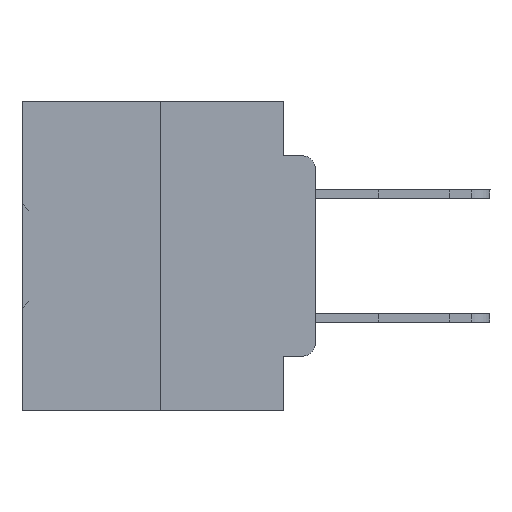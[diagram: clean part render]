
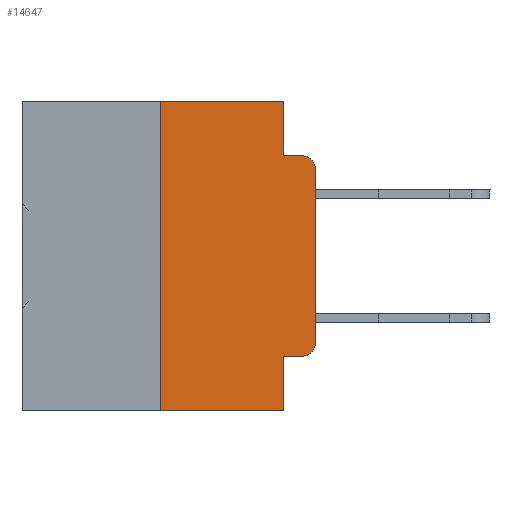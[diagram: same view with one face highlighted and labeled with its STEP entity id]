
A CAD part, left-side view. The second image highlights one B-rep face of the part: STEP entity #14647.
In plain terms, the highlighted planar face has unit normal (-1, 0, 0).
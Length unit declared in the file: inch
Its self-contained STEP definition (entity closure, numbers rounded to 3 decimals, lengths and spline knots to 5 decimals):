
#165 = ORIENTED_EDGE ( 'NONE', *, *, #10453, .F. ) ;
#388 = LINE ( 'NONE', #12724, #21902 ) ;
#482 = CARTESIAN_POINT ( 'NONE',  ( 0., 0.02, -0.3915 ) ) ;
#504 = EDGE_CURVE ( 'NONE', #18739, #6508, #18094, .T. ) ;
#889 = DIRECTION ( 'NONE',  ( 0., 0., -1. ) ) ;
#1047 = CARTESIAN_POINT ( 'NONE',  ( 0., 0.473, 0. ) ) ;
#1151 = VERTEX_POINT ( 'NONE', #35443 ) ;
#1273 = CARTESIAN_POINT ( 'NONE',  ( 0., 0.25, -0.5 ) ) ;
#1347 = VECTOR ( 'NONE', #1844, 39.37008 ) ;
#1844 = DIRECTION ( 'NONE',  ( 0., 0., 1. ) ) ;
#3006 = ORIENTED_EDGE ( 'NONE', *, *, #504, .T. ) ;
#3574 = VERTEX_POINT ( 'NONE', #27225 ) ;
#3698 = ORIENTED_EDGE ( 'NONE', *, *, #39091, .F. ) ;
#4231 = EDGE_CURVE ( 'NONE', #32129, #24944, #15705, .T. ) ;
#4873 = DIRECTION ( 'NONE',  ( 0., -1., 0. ) ) ;
#4876 = EDGE_CURVE ( 'NONE', #31318, #14479, #19327, .T. ) ;
#5025 = CARTESIAN_POINT ( 'NONE',  ( 0., 0., 0. ) ) ;
#5856 = DIRECTION ( 'NONE',  ( 0., 0., 1. ) ) ;
#6166 = ORIENTED_EDGE ( 'NONE', *, *, #20679, .T. ) ;
#6465 = VECTOR ( 'NONE', #28277, 39.37008 ) ;
#6508 = VERTEX_POINT ( 'NONE', #35220 ) ;
#6914 = LINE ( 'NONE', #37143, #18299 ) ;
#6916 = ORIENTED_EDGE ( 'NONE', *, *, #4231, .T. ) ;
#7059 = AXIS2_PLACEMENT_3D ( 'NONE', #482, #12627, #889 ) ;
#8066 = DIRECTION ( 'NONE',  ( 0., 0., -1. ) ) ;
#9365 = EDGE_CURVE ( 'NONE', #18739, #26156, #39066, .T. ) ;
#9749 = ORIENTED_EDGE ( 'NONE', *, *, #16248, .T. ) ;
#10453 = EDGE_CURVE ( 'NONE', #26156, #31318, #14223, .T. ) ;
#10498 = ORIENTED_EDGE ( 'NONE', *, *, #12105, .T. ) ;
#10657 = CARTESIAN_POINT ( 'NONE',  ( 0., 0.02, -0.1085 ) ) ;
#12105 = EDGE_CURVE ( 'NONE', #18230, #3574, #24518, .T. ) ;
#12390 = ORIENTED_EDGE ( 'NONE', *, *, #9365, .F. ) ;
#12627 = DIRECTION ( 'NONE',  ( -1., 0., 0. ) ) ;
#12724 = CARTESIAN_POINT ( 'NONE',  ( 0., 0.051, -0.0885 ) ) ;
#13373 = DIRECTION ( 'NONE',  ( 0., 0., -1. ) ) ;
#13827 = DIRECTION ( 'NONE',  ( -1., 0., 0. ) ) ;
#14223 = LINE ( 'NONE', #17402, #26185 ) ;
#14479 = VERTEX_POINT ( 'NONE', #38268 ) ;
#14643 = CARTESIAN_POINT ( 'NONE',  ( 0., 0., -0.1085 ) ) ;
#14647 = ADVANCED_FACE ( 'NONE', ( #28486 ), #30913, .F. ) ;
#14723 = CARTESIAN_POINT ( 'NONE',  ( 0., 0.051, -0.4115 ) ) ;
#15300 = CARTESIAN_POINT ( 'NONE',  ( 0., 0.473, -0.5 ) ) ;
#15705 = CIRCLE ( 'NONE', #37927, 0.02 ) ;
#16248 = EDGE_CURVE ( 'NONE', #1151, #32129, #34682, .T. ) ;
#16337 = CARTESIAN_POINT ( 'NONE',  ( 0., 0.051, 0. ) ) ;
#16974 = VECTOR ( 'NONE', #18554, 39.37008 ) ;
#17402 = CARTESIAN_POINT ( 'NONE',  ( 0., 0.473, 0. ) ) ;
#17469 = VECTOR ( 'NONE', #5856, 39.37008 ) ;
#18094 = LINE ( 'NONE', #15300, #38272 ) ;
#18230 = VERTEX_POINT ( 'NONE', #14723 ) ;
#18299 = VECTOR ( 'NONE', #28201, 39.37008 ) ;
#18324 = CARTESIAN_POINT ( 'NONE',  ( 0., 0.051, 0. ) ) ;
#18554 = DIRECTION ( 'NONE',  ( 0., -1., 0. ) ) ;
#18739 = VERTEX_POINT ( 'NONE', #1273 ) ;
#19148 = DIRECTION ( 'NONE',  ( 1., 0., 0. ) ) ;
#19206 = EDGE_LOOP ( 'NONE', ( #9749, #6916, #25173, #22682, #165, #12390, #3006, #3698, #10498, #6166 ) ) ;
#19327 = LINE ( 'NONE', #16337, #6465 ) ;
#20679 = EDGE_CURVE ( 'NONE', #3574, #1151, #37539, .T. ) ;
#20772 = CARTESIAN_POINT ( 'NONE',  ( 0., 0.25, 0. ) ) ;
#21902 = VECTOR ( 'NONE', #31030, 39.37008 ) ;
#22682 = ORIENTED_EDGE ( 'NONE', *, *, #4876, .F. ) ;
#24518 = LINE ( 'NONE', #33673, #16974 ) ;
#24944 = VERTEX_POINT ( 'NONE', #36343 ) ;
#25173 = ORIENTED_EDGE ( 'NONE', *, *, #35511, .F. ) ;
#26156 = VERTEX_POINT ( 'NONE', #29074 ) ;
#26185 = VECTOR ( 'NONE', #4873, 39.37008 ) ;
#27225 = CARTESIAN_POINT ( 'NONE',  ( 0., 0.02, -0.4115 ) ) ;
#28201 = DIRECTION ( 'NONE',  ( 0., 0., -1. ) ) ;
#28277 = DIRECTION ( 'NONE',  ( 0., 0., -1. ) ) ;
#28486 = FACE_OUTER_BOUND ( 'NONE', #19206, .T. ) ;
#29074 = CARTESIAN_POINT ( 'NONE',  ( 0., 0.25, 0. ) ) ;
#30913 = PLANE ( 'NONE',  #34287 ) ;
#31030 = DIRECTION ( 'NONE',  ( 0., -1., 0. ) ) ;
#31318 = VERTEX_POINT ( 'NONE', #18324 ) ;
#32129 = VERTEX_POINT ( 'NONE', #14643 ) ;
#33673 = CARTESIAN_POINT ( 'NONE',  ( 0., 0.051, -0.4115 ) ) ;
#34287 = AXIS2_PLACEMENT_3D ( 'NONE', #1047, #19148, #13373 ) ;
#34682 = LINE ( 'NONE', #5025, #1347 ) ;
#35220 = CARTESIAN_POINT ( 'NONE',  ( 0., 0.051, -0.5 ) ) ;
#35443 = CARTESIAN_POINT ( 'NONE',  ( 0., 0., -0.3915 ) ) ;
#35511 = EDGE_CURVE ( 'NONE', #14479, #24944, #388, .T. ) ;
#36343 = CARTESIAN_POINT ( 'NONE',  ( 0., 0.02, -0.0885 ) ) ;
#37143 = CARTESIAN_POINT ( 'NONE',  ( 0., 0.051, 0. ) ) ;
#37163 = DIRECTION ( 'NONE',  ( 0., -1., 0. ) ) ;
#37539 = CIRCLE ( 'NONE', #7059, 0.02 ) ;
#37927 = AXIS2_PLACEMENT_3D ( 'NONE', #10657, #13827, #8066 ) ;
#38268 = CARTESIAN_POINT ( 'NONE',  ( 0., 0.051, -0.0885 ) ) ;
#38272 = VECTOR ( 'NONE', #37163, 39.37008 ) ;
#39066 = LINE ( 'NONE', #20772, #17469 ) ;
#39091 = EDGE_CURVE ( 'NONE', #18230, #6508, #6914, .T. ) ;
